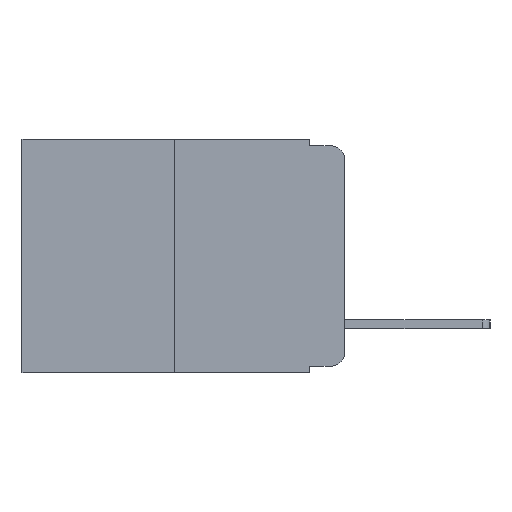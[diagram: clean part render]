
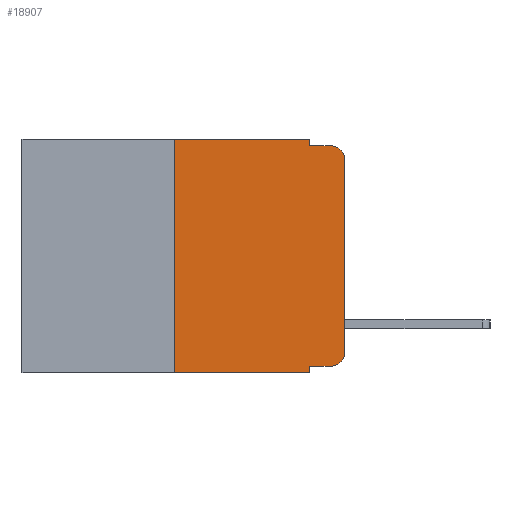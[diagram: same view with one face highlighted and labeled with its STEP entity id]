
A CAD part, left-side view. The second image highlights one B-rep face of the part: STEP entity #18907.
In plain terms, the highlighted planar face has unit normal (-1, 0, 0).
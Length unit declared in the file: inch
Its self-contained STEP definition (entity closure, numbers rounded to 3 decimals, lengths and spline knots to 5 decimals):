
#154 = AXIS2_PLACEMENT_3D ( 'NONE', #18492, #18688, #18664 ) ;
#469 = DIRECTION ( 'NONE',  ( 0., 0., -1. ) ) ;
#903 = EDGE_CURVE ( 'NONE', #6022, #9544, #12432, .T. ) ;
#924 = VECTOR ( 'NONE', #7602, 39.37008 ) ;
#989 = VERTEX_POINT ( 'NONE', #2804 ) ;
#1064 = EDGE_CURVE ( 'NONE', #989, #16834, #13328, .T. ) ;
#1203 = DIRECTION ( 'NONE',  ( -1., 0., 0. ) ) ;
#1853 = DIRECTION ( 'NONE',  ( 0., 0., -1. ) ) ;
#2001 = ORIENTED_EDGE ( 'NONE', *, *, #7372, .F. ) ;
#2237 = CARTESIAN_POINT ( 'NONE',  ( 0., 0.25, 0. ) ) ;
#2312 = ORIENTED_EDGE ( 'NONE', *, *, #12582, .F. ) ;
#2382 = VECTOR ( 'NONE', #14196, 39.37008 ) ;
#2804 = CARTESIAN_POINT ( 'NONE',  ( 0., 0.051, 0. ) ) ;
#3079 = CARTESIAN_POINT ( 'NONE',  ( 0., 0.02, -0.01 ) ) ;
#3631 = CARTESIAN_POINT ( 'NONE',  ( 0., 0.051, -0.01 ) ) ;
#3646 = DIRECTION ( 'NONE',  ( 0., 0., 1. ) ) ;
#4331 = CARTESIAN_POINT ( 'NONE',  ( 0., 0.051, 0. ) ) ;
#4471 = LINE ( 'NONE', #4331, #23793 ) ;
#5672 = CARTESIAN_POINT ( 'NONE',  ( 0., 0., 0. ) ) ;
#5810 = VERTEX_POINT ( 'NONE', #20676 ) ;
#5820 = AXIS2_PLACEMENT_3D ( 'NONE', #12679, #1203, #14552 ) ;
#5949 = EDGE_CURVE ( 'NONE', #18251, #5810, #6575, .T. ) ;
#6022 = VERTEX_POINT ( 'NONE', #16778 ) ;
#6575 = CIRCLE ( 'NONE', #154, 0.02 ) ;
#6950 = VERTEX_POINT ( 'NONE', #18929 ) ;
#7372 = EDGE_CURVE ( 'NONE', #9544, #989, #17433, .T. ) ;
#7582 = EDGE_CURVE ( 'NONE', #6022, #8410, #7818, .T. ) ;
#7599 = PLANE ( 'NONE',  #17813 ) ;
#7602 = DIRECTION ( 'NONE',  ( 0., 0., 1. ) ) ;
#7818 = LINE ( 'NONE', #16150, #22130 ) ;
#8302 = VECTOR ( 'NONE', #23555, 39.37008 ) ;
#8410 = VERTEX_POINT ( 'NONE', #9641 ) ;
#8508 = EDGE_LOOP ( 'NONE', ( #19116, #20300, #13040, #23452, #2001, #17635, #16184, #2312, #9817, #16831 ) ) ;
#9544 = VERTEX_POINT ( 'NONE', #24031 ) ;
#9641 = CARTESIAN_POINT ( 'NONE',  ( 0., 0.051, -0.343 ) ) ;
#9817 = ORIENTED_EDGE ( 'NONE', *, *, #24025, .T. ) ;
#10002 = VERTEX_POINT ( 'NONE', #17921 ) ;
#11432 = CARTESIAN_POINT ( 'NONE',  ( 0., 0.051, -0.01 ) ) ;
#11882 = CIRCLE ( 'NONE', #5820, 0.02 ) ;
#12432 = LINE ( 'NONE', #2237, #22890 ) ;
#12582 = EDGE_CURVE ( 'NONE', #10002, #8410, #4471, .T. ) ;
#12679 = CARTESIAN_POINT ( 'NONE',  ( 0., 0.02, -0.03 ) ) ;
#12780 = CARTESIAN_POINT ( 'NONE',  ( 0., 0.051, 0. ) ) ;
#12850 = CARTESIAN_POINT ( 'NONE',  ( 0., 0.051, -0.333 ) ) ;
#13040 = ORIENTED_EDGE ( 'NONE', *, *, #23478, .F. ) ;
#13291 = DIRECTION ( 'NONE',  ( 1., 0., 0. ) ) ;
#13328 = LINE ( 'NONE', #12780, #8302 ) ;
#13354 = EDGE_CURVE ( 'NONE', #6950, #21226, #11882, .T. ) ;
#14196 = DIRECTION ( 'NONE',  ( 0., -1., 0. ) ) ;
#14552 = DIRECTION ( 'NONE',  ( 0., 0., -1. ) ) ;
#14859 = VECTOR ( 'NONE', #14981, 39.37008 ) ;
#14981 = DIRECTION ( 'NONE',  ( 0., -1., 0. ) ) ;
#15962 = CARTESIAN_POINT ( 'NONE',  ( 0., 0.473, 0. ) ) ;
#16150 = CARTESIAN_POINT ( 'NONE',  ( 0., 0.473, -0.343 ) ) ;
#16184 = ORIENTED_EDGE ( 'NONE', *, *, #7582, .T. ) ;
#16778 = CARTESIAN_POINT ( 'NONE',  ( 0., 0.25, -0.343 ) ) ;
#16831 = ORIENTED_EDGE ( 'NONE', *, *, #5949, .T. ) ;
#16834 = VERTEX_POINT ( 'NONE', #11432 ) ;
#17090 = FACE_OUTER_BOUND ( 'NONE', #8508, .T. ) ;
#17433 = LINE ( 'NONE', #15962, #2382 ) ;
#17635 = ORIENTED_EDGE ( 'NONE', *, *, #903, .F. ) ;
#17813 = AXIS2_PLACEMENT_3D ( 'NONE', #18713, #13291, #1853 ) ;
#17921 = CARTESIAN_POINT ( 'NONE',  ( 0., 0.051, -0.333 ) ) ;
#18028 = DIRECTION ( 'NONE',  ( 0., -1., 0. ) ) ;
#18251 = VERTEX_POINT ( 'NONE', #21270 ) ;
#18492 = CARTESIAN_POINT ( 'NONE',  ( 0., 0.02, -0.313 ) ) ;
#18513 = VECTOR ( 'NONE', #22111, 39.37008 ) ;
#18664 = DIRECTION ( 'NONE',  ( 0., 0., -1. ) ) ;
#18688 = DIRECTION ( 'NONE',  ( -1., 0., 0. ) ) ;
#18713 = CARTESIAN_POINT ( 'NONE',  ( 0., 0.473, 0. ) ) ;
#18907 = ADVANCED_FACE ( 'NONE', ( #17090 ), #7599, .F. ) ;
#18929 = CARTESIAN_POINT ( 'NONE',  ( 0., 0., -0.03 ) ) ;
#19104 = LINE ( 'NONE', #12850, #18513 ) ;
#19116 = ORIENTED_EDGE ( 'NONE', *, *, #21774, .T. ) ;
#19230 = LINE ( 'NONE', #3631, #14859 ) ;
#20300 = ORIENTED_EDGE ( 'NONE', *, *, #13354, .T. ) ;
#20676 = CARTESIAN_POINT ( 'NONE',  ( 0., 0., -0.313 ) ) ;
#21074 = LINE ( 'NONE', #5672, #924 ) ;
#21226 = VERTEX_POINT ( 'NONE', #3079 ) ;
#21270 = CARTESIAN_POINT ( 'NONE',  ( 0., 0.02, -0.333 ) ) ;
#21774 = EDGE_CURVE ( 'NONE', #5810, #6950, #21074, .T. ) ;
#22111 = DIRECTION ( 'NONE',  ( 0., -1., 0. ) ) ;
#22130 = VECTOR ( 'NONE', #18028, 39.37008 ) ;
#22890 = VECTOR ( 'NONE', #3646, 39.37008 ) ;
#23452 = ORIENTED_EDGE ( 'NONE', *, *, #1064, .F. ) ;
#23478 = EDGE_CURVE ( 'NONE', #16834, #21226, #19230, .T. ) ;
#23555 = DIRECTION ( 'NONE',  ( 0., 0., -1. ) ) ;
#23793 = VECTOR ( 'NONE', #469, 39.37008 ) ;
#24025 = EDGE_CURVE ( 'NONE', #10002, #18251, #19104, .T. ) ;
#24031 = CARTESIAN_POINT ( 'NONE',  ( 0., 0.25, 0. ) ) ;
